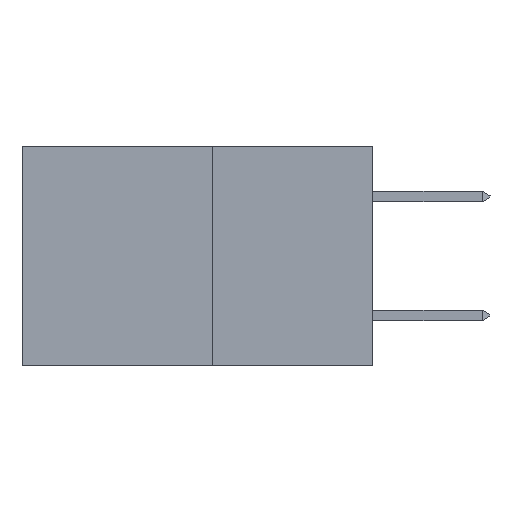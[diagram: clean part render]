
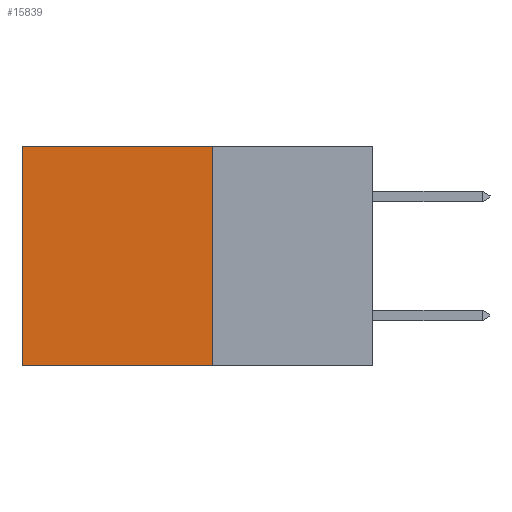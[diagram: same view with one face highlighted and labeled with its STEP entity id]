
A CAD part, left-side view. The second image highlights one B-rep face of the part: STEP entity #15839.
In plain terms, the highlighted planar face has unit normal (-1, 0, 0).
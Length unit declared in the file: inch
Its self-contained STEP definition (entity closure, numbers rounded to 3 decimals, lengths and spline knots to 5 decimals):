
#142 = DIRECTION ( 'NONE',  ( 0., 1., 0. ) ) ;
#1592 = DIRECTION ( 'NONE',  ( 0., 0., -1. ) ) ;
#1750 = DIRECTION ( 'NONE',  ( 0., 0., -1. ) ) ;
#3246 = EDGE_CURVE ( 'NONE', #8876, #14842, #34035, .T. ) ;
#3792 = EDGE_CURVE ( 'NONE', #24317, #14842, #14102, .T. ) ;
#4334 = ORIENTED_EDGE ( 'NONE', *, *, #15411, .T. ) ;
#6176 = ORIENTED_EDGE ( 'NONE', *, *, #3246, .F. ) ;
#7104 = VECTOR ( 'NONE', #13872, 39.37008 ) ;
#7924 = CARTESIAN_POINT ( 'NONE',  ( 0.277, 0.27, 0. ) ) ;
#8698 = CARTESIAN_POINT ( 'NONE',  ( 0.277, 0.59, -0.37 ) ) ;
#8876 = VERTEX_POINT ( 'NONE', #23357 ) ;
#10763 = LINE ( 'NONE', #17618, #31861 ) ;
#13872 = DIRECTION ( 'NONE',  ( 0., 0., -1. ) ) ;
#14102 = LINE ( 'NONE', #8698, #7104 ) ;
#14842 = VERTEX_POINT ( 'NONE', #24455 ) ;
#15113 = EDGE_CURVE ( 'NONE', #31306, #8876, #10763, .T. ) ;
#15411 = EDGE_CURVE ( 'NONE', #31306, #24317, #23557, .T. ) ;
#15839 = ADVANCED_FACE ( 'NONE', ( #23528 ), #30658, .F. ) ;
#16509 = VECTOR ( 'NONE', #18404, 39.37008 ) ;
#17448 = DIRECTION ( 'NONE',  ( 1., 0., 0. ) ) ;
#17618 = CARTESIAN_POINT ( 'NONE',  ( 0.277, 0.27, -0.37 ) ) ;
#18404 = DIRECTION ( 'NONE',  ( 0., 1., 0. ) ) ;
#21460 = ORIENTED_EDGE ( 'NONE', *, *, #3792, .T. ) ;
#21625 = CARTESIAN_POINT ( 'NONE',  ( 0.277, 0.27, 0. ) ) ;
#23002 = AXIS2_PLACEMENT_3D ( 'NONE', #33311, #17448, #1592 ) ;
#23357 = CARTESIAN_POINT ( 'NONE',  ( 0.277, 0.27, -0.37 ) ) ;
#23526 = CARTESIAN_POINT ( 'NONE',  ( 0.277, 0.27, -0.37 ) ) ;
#23528 = FACE_OUTER_BOUND ( 'NONE', #31076, .T. ) ;
#23557 = LINE ( 'NONE', #7924, #16509 ) ;
#24253 = ORIENTED_EDGE ( 'NONE', *, *, #15113, .F. ) ;
#24317 = VERTEX_POINT ( 'NONE', #33998 ) ;
#24455 = CARTESIAN_POINT ( 'NONE',  ( 0.277, 0.59, -0.37 ) ) ;
#26992 = VECTOR ( 'NONE', #142, 39.37008 ) ;
#30658 = PLANE ( 'NONE',  #23002 ) ;
#31076 = EDGE_LOOP ( 'NONE', ( #21460, #6176, #24253, #4334 ) ) ;
#31306 = VERTEX_POINT ( 'NONE', #21625 ) ;
#31861 = VECTOR ( 'NONE', #1750, 39.37008 ) ;
#33311 = CARTESIAN_POINT ( 'NONE',  ( 0.277, 0.27, -0.37 ) ) ;
#33998 = CARTESIAN_POINT ( 'NONE',  ( 0.277, 0.59, 0. ) ) ;
#34035 = LINE ( 'NONE', #23526, #26992 ) ;
